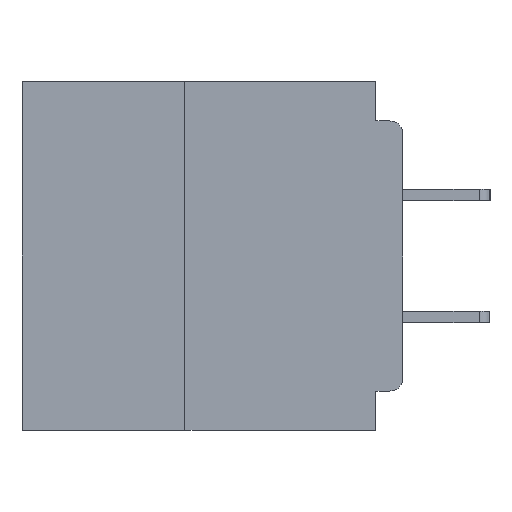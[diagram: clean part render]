
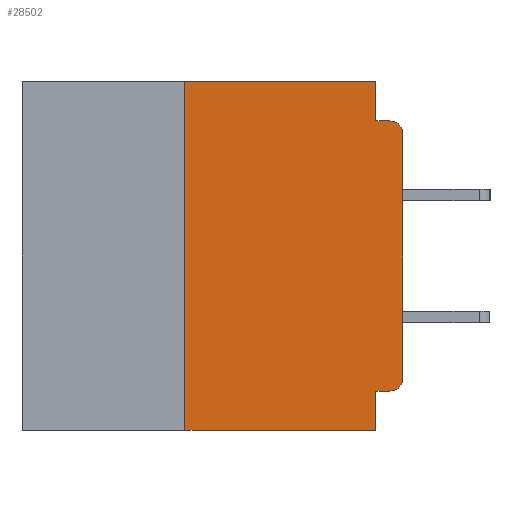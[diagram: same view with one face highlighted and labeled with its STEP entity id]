
A CAD part, left-side view. The second image highlights one B-rep face of the part: STEP entity #28502.
In plain terms, the highlighted planar face has unit normal (-1, 0, 0).
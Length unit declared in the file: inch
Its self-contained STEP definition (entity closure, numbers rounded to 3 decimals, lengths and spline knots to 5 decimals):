
#180 = VERTEX_POINT ( 'NONE', #43453 ) ;
#736 = CARTESIAN_POINT ( 'NONE',  ( 0., 0., 0. ) ) ;
#918 = LINE ( 'NONE', #34739, #9941 ) ;
#3378 = PLANE ( 'NONE',  #14263 ) ;
#3609 = FACE_OUTER_BOUND ( 'NONE', #4463, .T. ) ;
#3848 = ORIENTED_EDGE ( 'NONE', *, *, #27503, .F. ) ;
#4463 = EDGE_LOOP ( 'NONE', ( #19001, #23494, #27318, #18177, #3848, #19222, #47216, #41704, #16250, #31832 ) ) ;
#4511 = CARTESIAN_POINT ( 'NONE',  ( 0., 0.031, 0. ) ) ;
#7259 = DIRECTION ( 'NONE',  ( 1., 0., 0. ) ) ;
#8706 = DIRECTION ( 'NONE',  ( 0., -1., 0. ) ) ;
#9635 = VERTEX_POINT ( 'NONE', #35185 ) ;
#9941 = VECTOR ( 'NONE', #38520, 39.37008 ) ;
#10854 = VECTOR ( 'NONE', #12007, 39.37008 ) ;
#11419 = VECTOR ( 'NONE', #12462, 39.37008 ) ;
#12007 = DIRECTION ( 'NONE',  ( 0., -1., 0. ) ) ;
#12328 = CARTESIAN_POINT ( 'NONE',  ( 0., 0.25, 0. ) ) ;
#12351 = DIRECTION ( 'NONE',  ( 0., 1., 0. ) ) ;
#12462 = DIRECTION ( 'NONE',  ( 0., -1., 0. ) ) ;
#13180 = CARTESIAN_POINT ( 'NONE',  ( 0., 0., -0.34 ) ) ;
#13554 = EDGE_CURVE ( 'NONE', #180, #42205, #42249, .T. ) ;
#13727 = VECTOR ( 'NONE', #47362, 39.37008 ) ;
#14002 = CARTESIAN_POINT ( 'NONE',  ( 0., 0., -0.06 ) ) ;
#14226 = CARTESIAN_POINT ( 'NONE',  ( 0., 0.015, -0.045 ) ) ;
#14263 = AXIS2_PLACEMENT_3D ( 'NONE', #40957, #7259, #33562 ) ;
#14883 = LINE ( 'NONE', #43618, #13727 ) ;
#15191 = LINE ( 'NONE', #40397, #23969 ) ;
#15801 = CARTESIAN_POINT ( 'NONE',  ( 0., 0., -0.355 ) ) ;
#16185 = LINE ( 'NONE', #31172, #26114 ) ;
#16250 = ORIENTED_EDGE ( 'NONE', *, *, #13554, .F. ) ;
#16313 = EDGE_CURVE ( 'NONE', #36938, #9635, #20249, .T. ) ;
#17219 = CARTESIAN_POINT ( 'NONE',  ( 0., 0.25, -0.4 ) ) ;
#17918 = DIRECTION ( 'NONE',  ( 0., 0., -1. ) ) ;
#18177 = ORIENTED_EDGE ( 'NONE', *, *, #43490, .F. ) ;
#18314 = CIRCLE ( 'NONE', #40197, 0.015 ) ;
#19001 = ORIENTED_EDGE ( 'NONE', *, *, #37304, .T. ) ;
#19222 = ORIENTED_EDGE ( 'NONE', *, *, #46723, .F. ) ;
#19339 = CARTESIAN_POINT ( 'NONE',  ( 0., 0.031, -0.045 ) ) ;
#19467 = DIRECTION ( 'NONE',  ( -1., 0., 0. ) ) ;
#20249 = LINE ( 'NONE', #31151, #11419 ) ;
#21113 = DIRECTION ( 'NONE',  ( -1., 0., 0. ) ) ;
#22231 = VECTOR ( 'NONE', #27155, 39.37008 ) ;
#23494 = ORIENTED_EDGE ( 'NONE', *, *, #33944, .T. ) ;
#23969 = VECTOR ( 'NONE', #17918, 39.37008 ) ;
#25904 = VERTEX_POINT ( 'NONE', #19339 ) ;
#26114 = VECTOR ( 'NONE', #8706, 39.37008 ) ;
#26204 = VERTEX_POINT ( 'NONE', #14226 ) ;
#26797 = VERTEX_POINT ( 'NONE', #4511 ) ;
#27155 = DIRECTION ( 'NONE',  ( 0., 0., 1. ) ) ;
#27318 = ORIENTED_EDGE ( 'NONE', *, *, #31398, .F. ) ;
#27503 = EDGE_CURVE ( 'NONE', #33110, #26797, #16185, .T. ) ;
#27575 = CARTESIAN_POINT ( 'NONE',  ( 0., 0.031, -0.355 ) ) ;
#28502 = ADVANCED_FACE ( 'NONE', ( #3609 ), #3378, .F. ) ;
#29005 = VERTEX_POINT ( 'NONE', #14002 ) ;
#29149 = CIRCLE ( 'NONE', #39926, 0.015 ) ;
#29321 = EDGE_CURVE ( 'NONE', #42205, #9635, #15191, .T. ) ;
#29927 = VECTOR ( 'NONE', #12351, 39.37008 ) ;
#30835 = LINE ( 'NONE', #38265, #10854 ) ;
#31039 = LINE ( 'NONE', #736, #22231 ) ;
#31151 = CARTESIAN_POINT ( 'NONE',  ( 0., 0.437, -0.4 ) ) ;
#31172 = CARTESIAN_POINT ( 'NONE',  ( 0., 0.437, 0. ) ) ;
#31398 = EDGE_CURVE ( 'NONE', #25904, #26204, #30835, .T. ) ;
#31832 = ORIENTED_EDGE ( 'NONE', *, *, #38534, .T. ) ;
#33110 = VERTEX_POINT ( 'NONE', #12328 ) ;
#33562 = DIRECTION ( 'NONE',  ( 0., 0., -1. ) ) ;
#33944 = EDGE_CURVE ( 'NONE', #29005, #26204, #18314, .T. ) ;
#34739 = CARTESIAN_POINT ( 'NONE',  ( 0., 0.031, 0. ) ) ;
#35185 = CARTESIAN_POINT ( 'NONE',  ( 0., 0.031, -0.4 ) ) ;
#36938 = VERTEX_POINT ( 'NONE', #17219 ) ;
#37304 = EDGE_CURVE ( 'NONE', #38777, #29005, #31039, .T. ) ;
#38265 = CARTESIAN_POINT ( 'NONE',  ( 0., 0., -0.045 ) ) ;
#38520 = DIRECTION ( 'NONE',  ( 0., 0., -1. ) ) ;
#38534 = EDGE_CURVE ( 'NONE', #180, #38777, #29149, .T. ) ;
#38777 = VERTEX_POINT ( 'NONE', #13180 ) ;
#39926 = AXIS2_PLACEMENT_3D ( 'NONE', #41891, #19467, #45693 ) ;
#40197 = AXIS2_PLACEMENT_3D ( 'NONE', #43580, #21113, #47329 ) ;
#40397 = CARTESIAN_POINT ( 'NONE',  ( 0., 0.031, -0.4 ) ) ;
#40957 = CARTESIAN_POINT ( 'NONE',  ( 0., 0.437, 0. ) ) ;
#41704 = ORIENTED_EDGE ( 'NONE', *, *, #29321, .F. ) ;
#41891 = CARTESIAN_POINT ( 'NONE',  ( 0., 0.015, -0.34 ) ) ;
#42205 = VERTEX_POINT ( 'NONE', #27575 ) ;
#42249 = LINE ( 'NONE', #15801, #29927 ) ;
#43453 = CARTESIAN_POINT ( 'NONE',  ( 0., 0.015, -0.355 ) ) ;
#43490 = EDGE_CURVE ( 'NONE', #26797, #25904, #918, .T. ) ;
#43580 = CARTESIAN_POINT ( 'NONE',  ( 0., 0.015, -0.06 ) ) ;
#43618 = CARTESIAN_POINT ( 'NONE',  ( 0., 0.25, -0.4 ) ) ;
#45693 = DIRECTION ( 'NONE',  ( 0., 0., -1. ) ) ;
#46723 = EDGE_CURVE ( 'NONE', #36938, #33110, #14883, .T. ) ;
#47216 = ORIENTED_EDGE ( 'NONE', *, *, #16313, .T. ) ;
#47329 = DIRECTION ( 'NONE',  ( 0., 0., -1. ) ) ;
#47362 = DIRECTION ( 'NONE',  ( 0., 0., 1. ) ) ;
